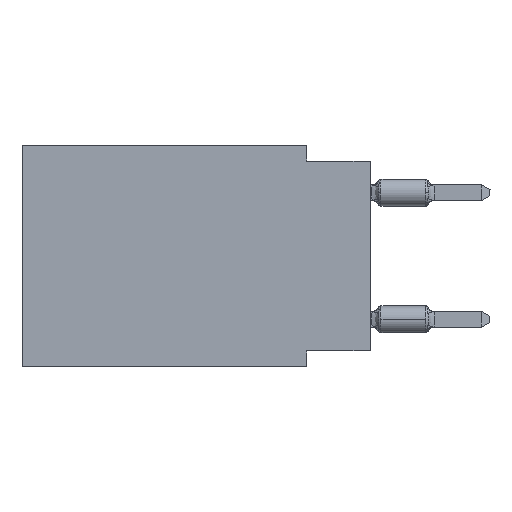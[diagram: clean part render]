
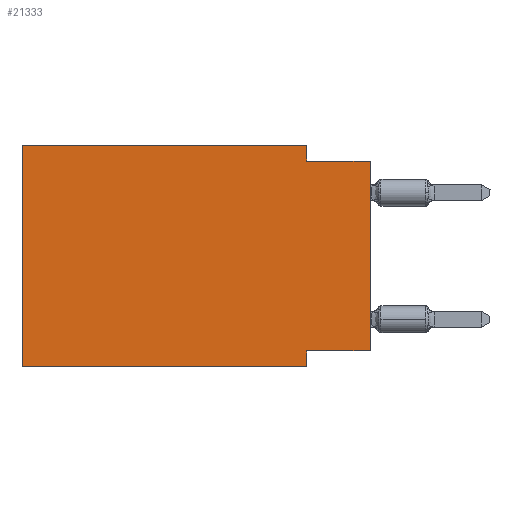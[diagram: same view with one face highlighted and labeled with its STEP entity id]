
A CAD part, left-side view. The second image highlights one B-rep face of the part: STEP entity #21333.
In plain terms, the highlighted planar face has unit normal (-1, 0, 0).
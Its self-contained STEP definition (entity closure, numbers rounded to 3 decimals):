
#231 = ORIENTED_EDGE ( 'NONE', *, *, #29741, .F. ) ;
#908 = VECTOR ( 'NONE', #18868, 1000. ) ;
#1428 = CARTESIAN_POINT ( 'NONE',  ( 0., 13.97, 0. ) ) ;
#1536 = EDGE_CURVE ( 'NONE', #3796, #33474, #33114, .T. ) ;
#1671 = DIRECTION ( 'NONE',  ( 0., -1., 0. ) ) ;
#2999 = AXIS2_PLACEMENT_3D ( 'NONE', #24031, #32584, #43329 ) ;
#3015 = DIRECTION ( 'NONE',  ( 0., -1., 0. ) ) ;
#3426 = CARTESIAN_POINT ( 'NONE',  ( 0., 0., 0. ) ) ;
#3796 = VERTEX_POINT ( 'NONE', #31051 ) ;
#3869 = ORIENTED_EDGE ( 'NONE', *, *, #30957, .F. ) ;
#3884 = VECTOR ( 'NONE', #18359, 1000. ) ;
#4963 = EDGE_CURVE ( 'NONE', #40274, #33022, #18305, .T. ) ;
#6304 = ORIENTED_EDGE ( 'NONE', *, *, #4963, .T. ) ;
#7840 = CARTESIAN_POINT ( 'NONE',  ( 0., 13.97, 0. ) ) ;
#8439 = EDGE_CURVE ( 'NONE', #10105, #3796, #44839, .T. ) ;
#8532 = CARTESIAN_POINT ( 'NONE',  ( 0., 2.54, 0. ) ) ;
#8675 = VECTOR ( 'NONE', #3015, 1000. ) ;
#9257 = LINE ( 'NONE', #1428, #24484 ) ;
#9338 = CARTESIAN_POINT ( 'NONE',  ( 0., 2.54, -8.89 ) ) ;
#9951 = EDGE_LOOP ( 'NONE', ( #20048, #34581, #16121, #15821, #29799, #6304, #231, #3869 ) ) ;
#9967 = CARTESIAN_POINT ( 'NONE',  ( 0., 13.97, -8.89 ) ) ;
#10105 = VERTEX_POINT ( 'NONE', #8532 ) ;
#10304 = EDGE_CURVE ( 'NONE', #41399, #10105, #9257, .T. ) ;
#12745 = VECTOR ( 'NONE', #43968, 1000. ) ;
#13269 = FACE_OUTER_BOUND ( 'NONE', #9951, .T. ) ;
#14125 = CARTESIAN_POINT ( 'NONE',  ( 0., 2.54, -8.255 ) ) ;
#14174 = EDGE_CURVE ( 'NONE', #45536, #33474, #47934, .T. ) ;
#15821 = ORIENTED_EDGE ( 'NONE', *, *, #10304, .F. ) ;
#16121 = ORIENTED_EDGE ( 'NONE', *, *, #8439, .F. ) ;
#16693 = DIRECTION ( 'NONE',  ( 0., 0., -1. ) ) ;
#17182 = LINE ( 'NONE', #45800, #37582 ) ;
#17352 = CARTESIAN_POINT ( 'NONE',  ( 0., 0., -0.635 ) ) ;
#18305 = LINE ( 'NONE', #25168, #12745 ) ;
#18359 = DIRECTION ( 'NONE',  ( 0., 0., 1. ) ) ;
#18396 = LINE ( 'NONE', #7840, #908 ) ;
#18868 = DIRECTION ( 'NONE',  ( 0., 0., 1. ) ) ;
#20048 = ORIENTED_EDGE ( 'NONE', *, *, #14174, .T. ) ;
#21333 = ADVANCED_FACE ( 'NONE', ( #13269 ), #47000, .F. ) ;
#24031 = CARTESIAN_POINT ( 'NONE',  ( 0., 13.97, 0. ) ) ;
#24484 = VECTOR ( 'NONE', #1671, 1000. ) ;
#25168 = CARTESIAN_POINT ( 'NONE',  ( 0., 13.97, -8.89 ) ) ;
#25499 = VERTEX_POINT ( 'NONE', #14125 ) ;
#26898 = CARTESIAN_POINT ( 'NONE',  ( 0., 0., -8.255 ) ) ;
#29741 = EDGE_CURVE ( 'NONE', #25499, #33022, #17182, .T. ) ;
#29799 = ORIENTED_EDGE ( 'NONE', *, *, #29970, .F. ) ;
#29970 = EDGE_CURVE ( 'NONE', #40274, #41399, #18396, .T. ) ;
#30099 = VECTOR ( 'NONE', #41798, 1000. ) ;
#30957 = EDGE_CURVE ( 'NONE', #45536, #25499, #34232, .T. ) ;
#31051 = CARTESIAN_POINT ( 'NONE',  ( 0., 2.54, -0.635 ) ) ;
#31748 = CARTESIAN_POINT ( 'NONE',  ( 0., 13.97, 0. ) ) ;
#31790 = VECTOR ( 'NONE', #16693, 1000. ) ;
#32584 = DIRECTION ( 'NONE',  ( 1., 0., 0. ) ) ;
#33022 = VERTEX_POINT ( 'NONE', #9338 ) ;
#33114 = LINE ( 'NONE', #37262, #8675 ) ;
#33474 = VERTEX_POINT ( 'NONE', #17352 ) ;
#34232 = LINE ( 'NONE', #26898, #30099 ) ;
#34581 = ORIENTED_EDGE ( 'NONE', *, *, #1536, .F. ) ;
#34584 = CARTESIAN_POINT ( 'NONE',  ( 0., 0., -8.255 ) ) ;
#37262 = CARTESIAN_POINT ( 'NONE',  ( 0., 0., -0.635 ) ) ;
#37582 = VECTOR ( 'NONE', #42127, 1000. ) ;
#40274 = VERTEX_POINT ( 'NONE', #9967 ) ;
#41168 = CARTESIAN_POINT ( 'NONE',  ( 0., 2.54, 0. ) ) ;
#41399 = VERTEX_POINT ( 'NONE', #31748 ) ;
#41798 = DIRECTION ( 'NONE',  ( 0., 1., 0. ) ) ;
#42127 = DIRECTION ( 'NONE',  ( 0., 0., -1. ) ) ;
#43329 = DIRECTION ( 'NONE',  ( 0., 0., -1. ) ) ;
#43968 = DIRECTION ( 'NONE',  ( 0., -1., 0. ) ) ;
#44839 = LINE ( 'NONE', #41168, #31790 ) ;
#45536 = VERTEX_POINT ( 'NONE', #34584 ) ;
#45800 = CARTESIAN_POINT ( 'NONE',  ( 0., 2.54, -8.89 ) ) ;
#47000 = PLANE ( 'NONE',  #2999 ) ;
#47934 = LINE ( 'NONE', #3426, #3884 ) ;
